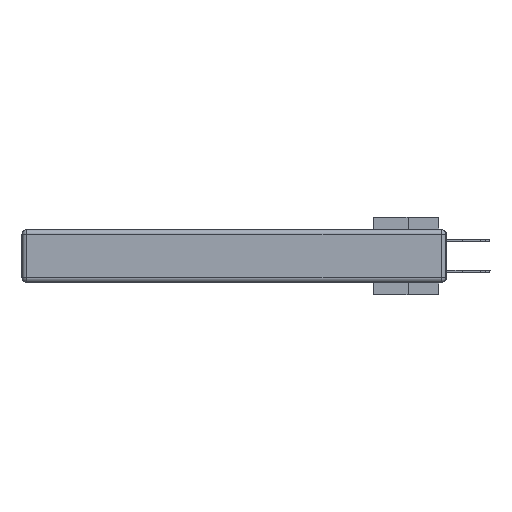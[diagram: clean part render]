
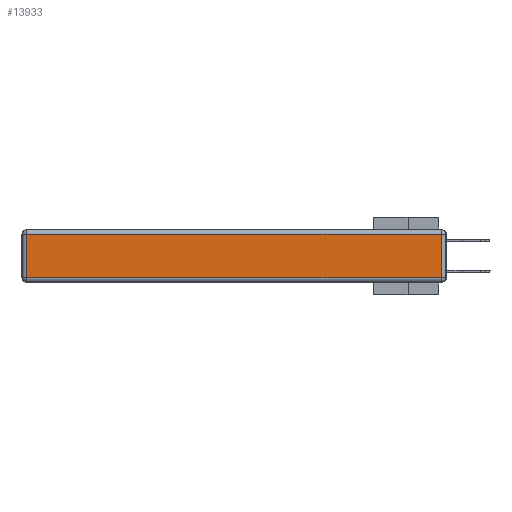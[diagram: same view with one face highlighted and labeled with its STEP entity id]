
A CAD part, left-side view. The second image highlights one B-rep face of the part: STEP entity #13933.
In plain terms, the highlighted planar face has unit normal (-1, 0, 0).
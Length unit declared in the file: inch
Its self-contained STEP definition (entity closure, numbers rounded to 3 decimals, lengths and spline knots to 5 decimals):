
#507 = ORIENTED_EDGE ( 'NONE', *, *, #40666, .T. ) ;
#630 = ORIENTED_EDGE ( 'NONE', *, *, #8015, .T. ) ;
#1200 = DIRECTION ( 'NONE',  ( 0., 0., 1. ) ) ;
#1614 = EDGE_CURVE ( 'NONE', #38410, #15939, #40835, .T. ) ;
#2153 = CARTESIAN_POINT ( 'NONE',  ( 0., 0.03, -0.313 ) ) ;
#3900 = DIRECTION ( 'NONE',  ( 0., -1., 0. ) ) ;
#4824 = EDGE_CURVE ( 'NONE', #15939, #35559, #7492, .T. ) ;
#5005 = AXIS2_PLACEMENT_3D ( 'NONE', #24310, #20741, #33593 ) ;
#7492 = LINE ( 'NONE', #10850, #23353 ) ;
#7998 = LINE ( 'NONE', #20867, #27624 ) ;
#8015 = EDGE_CURVE ( 'NONE', #35559, #26685, #17215, .T. ) ;
#8411 = CARTESIAN_POINT ( 'NONE',  ( 0., 2.72, -0.313 ) ) ;
#10850 = CARTESIAN_POINT ( 'NONE',  ( 0., 0., -0.313 ) ) ;
#11553 = VECTOR ( 'NONE', #1200, 39.37008 ) ;
#13933 = ADVANCED_FACE ( 'NONE', ( #40105 ), #30197, .T. ) ;
#14649 = ORIENTED_EDGE ( 'NONE', *, *, #4824, .T. ) ;
#14917 = DIRECTION ( 'NONE',  ( 0., 0., -1. ) ) ;
#15939 = VERTEX_POINT ( 'NONE', #8411 ) ;
#17215 = LINE ( 'NONE', #26483, #11553 ) ;
#20741 = DIRECTION ( 'NONE',  ( -1., 0., 0. ) ) ;
#20867 = CARTESIAN_POINT ( 'NONE',  ( 0., 2.75, -0.03 ) ) ;
#23353 = VECTOR ( 'NONE', #3900, 39.37008 ) ;
#24310 = CARTESIAN_POINT ( 'NONE',  ( 0., 0., -0.343 ) ) ;
#26391 = EDGE_LOOP ( 'NONE', ( #14649, #630, #507, #37094 ) ) ;
#26483 = CARTESIAN_POINT ( 'NONE',  ( 0., 0.03, -0.343 ) ) ;
#26685 = VERTEX_POINT ( 'NONE', #39937 ) ;
#27555 = CARTESIAN_POINT ( 'NONE',  ( 0., 2.72, -0.343 ) ) ;
#27624 = VECTOR ( 'NONE', #33720, 39.37008 ) ;
#30197 = PLANE ( 'NONE',  #5005 ) ;
#33593 = DIRECTION ( 'NONE',  ( 0., 0., 1. ) ) ;
#33720 = DIRECTION ( 'NONE',  ( 0., 1., 0. ) ) ;
#34431 = CARTESIAN_POINT ( 'NONE',  ( 0., 2.72, -0.03 ) ) ;
#35559 = VERTEX_POINT ( 'NONE', #2153 ) ;
#37094 = ORIENTED_EDGE ( 'NONE', *, *, #1614, .T. ) ;
#38410 = VERTEX_POINT ( 'NONE', #34431 ) ;
#39937 = CARTESIAN_POINT ( 'NONE',  ( 0., 0.03, -0.03 ) ) ;
#40105 = FACE_OUTER_BOUND ( 'NONE', #26391, .T. ) ;
#40666 = EDGE_CURVE ( 'NONE', #26685, #38410, #7998, .T. ) ;
#40800 = VECTOR ( 'NONE', #14917, 39.37008 ) ;
#40835 = LINE ( 'NONE', #27555, #40800 ) ;
